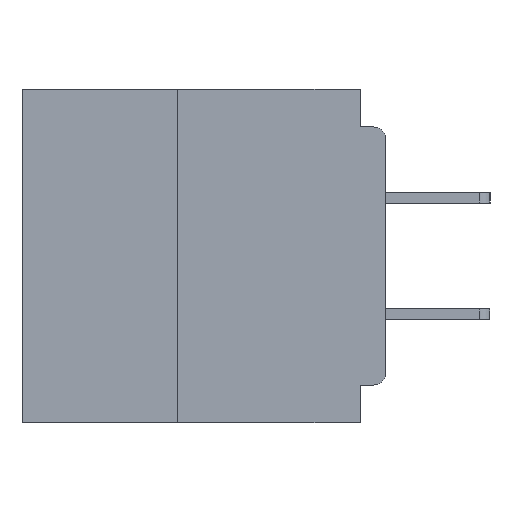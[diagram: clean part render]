
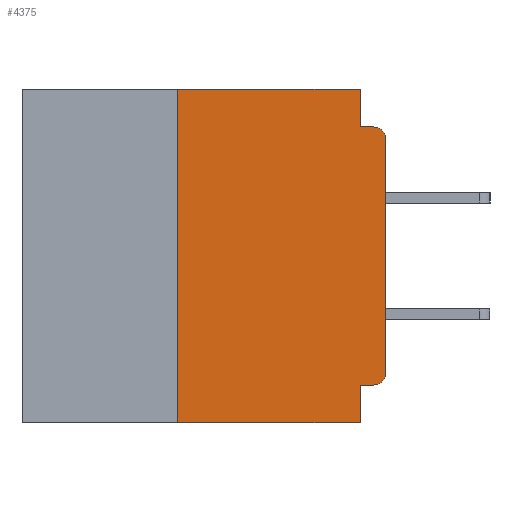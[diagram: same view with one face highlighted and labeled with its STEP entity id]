
A CAD part, left-side view. The second image highlights one B-rep face of the part: STEP entity #4375.
In plain terms, the highlighted planar face has unit normal (-1, 0, 0).
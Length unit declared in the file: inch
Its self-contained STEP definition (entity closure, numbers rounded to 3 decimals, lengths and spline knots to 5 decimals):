
#726 = EDGE_CURVE ( 'NONE', #33710, #32861, #31863, .T. ) ;
#844 = CIRCLE ( 'NONE', #5606, 0.015 ) ;
#1733 = DIRECTION ( 'NONE',  ( 0., -1., 0. ) ) ;
#3978 = CARTESIAN_POINT ( 'NONE',  ( 0., 0.031, 0. ) ) ;
#4185 = VECTOR ( 'NONE', #20784, 39.37008 ) ;
#4375 = ADVANCED_FACE ( 'NONE', ( #26787 ), #51676, .F. ) ;
#4654 = CARTESIAN_POINT ( 'NONE',  ( 0., 0., 0. ) ) ;
#4858 = DIRECTION ( 'NONE',  ( 0., 1., 0. ) ) ;
#5606 = AXIS2_PLACEMENT_3D ( 'NONE', #35649, #9319, #39950 ) ;
#5641 = ORIENTED_EDGE ( 'NONE', *, *, #44179, .F. ) ;
#5864 = CARTESIAN_POINT ( 'NONE',  ( 0., 0.015, -0.045 ) ) ;
#7448 = VERTEX_POINT ( 'NONE', #21349 ) ;
#7575 = CARTESIAN_POINT ( 'NONE',  ( 0., 0.015, -0.06 ) ) ;
#7986 = ORIENTED_EDGE ( 'NONE', *, *, #52729, .F. ) ;
#8077 = VECTOR ( 'NONE', #16363, 39.37008 ) ;
#8867 = VERTEX_POINT ( 'NONE', #40444 ) ;
#9319 = DIRECTION ( 'NONE',  ( -1., 0., 0. ) ) ;
#13557 = LINE ( 'NONE', #39957, #36845 ) ;
#13587 = DIRECTION ( 'NONE',  ( 0., 0., 1. ) ) ;
#13747 = VECTOR ( 'NONE', #1733, 39.37008 ) ;
#14950 = VERTEX_POINT ( 'NONE', #47479 ) ;
#16192 = CARTESIAN_POINT ( 'NONE',  ( 0., 0., -0.045 ) ) ;
#16347 = EDGE_LOOP ( 'NONE', ( #53151, #26699, #54415, #7986, #5641, #36179, #53733, #44092, #44790, #26195 ) ) ;
#16363 = DIRECTION ( 'NONE',  ( 0., -1., 0. ) ) ;
#16460 = CARTESIAN_POINT ( 'NONE',  ( 0., 0.015, -0.355 ) ) ;
#17698 = DIRECTION ( 'NONE',  ( 0., 0., -1. ) ) ;
#18506 = EDGE_CURVE ( 'NONE', #29937, #56159, #13557, .T. ) ;
#19112 = LINE ( 'NONE', #30955, #40934 ) ;
#19751 = LINE ( 'NONE', #34488, #41582 ) ;
#20784 = DIRECTION ( 'NONE',  ( 0., 0., -1. ) ) ;
#21035 = AXIS2_PLACEMENT_3D ( 'NONE', #7575, #27824, #17698 ) ;
#21349 = CARTESIAN_POINT ( 'NONE',  ( 0., 0.031, -0.4 ) ) ;
#23026 = CARTESIAN_POINT ( 'NONE',  ( 0., 0.25, 0. ) ) ;
#23324 = EDGE_CURVE ( 'NONE', #8867, #33710, #36530, .T. ) ;
#24668 = VECTOR ( 'NONE', #38396, 39.37008 ) ;
#26195 = ORIENTED_EDGE ( 'NONE', *, *, #51726, .T. ) ;
#26699 = ORIENTED_EDGE ( 'NONE', *, *, #726, .T. ) ;
#26787 = FACE_OUTER_BOUND ( 'NONE', #16347, .T. ) ;
#27824 = DIRECTION ( 'NONE',  ( -1., 0., 0. ) ) ;
#29469 = EDGE_CURVE ( 'NONE', #56159, #7448, #19112, .T. ) ;
#29937 = VERTEX_POINT ( 'NONE', #16460 ) ;
#30068 = DIRECTION ( 'NONE',  ( 0., 0., -1. ) ) ;
#30955 = CARTESIAN_POINT ( 'NONE',  ( 0., 0.031, -0.4 ) ) ;
#31863 = CIRCLE ( 'NONE', #21035, 0.015 ) ;
#32405 = EDGE_CURVE ( 'NONE', #50454, #7448, #55852, .T. ) ;
#32534 = VERTEX_POINT ( 'NONE', #3978 ) ;
#32861 = VERTEX_POINT ( 'NONE', #5864 ) ;
#33710 = VERTEX_POINT ( 'NONE', #51564 ) ;
#34488 = CARTESIAN_POINT ( 'NONE',  ( 0., 0.25, -0.4 ) ) ;
#35329 = DIRECTION ( 'NONE',  ( 0., 0., -1. ) ) ;
#35649 = CARTESIAN_POINT ( 'NONE',  ( 0., 0.015, -0.34 ) ) ;
#36179 = ORIENTED_EDGE ( 'NONE', *, *, #49793, .F. ) ;
#36285 = LINE ( 'NONE', #16192, #24668 ) ;
#36530 = LINE ( 'NONE', #4654, #45314 ) ;
#36845 = VECTOR ( 'NONE', #4858, 39.37008 ) ;
#38391 = LINE ( 'NONE', #45466, #13747 ) ;
#38396 = DIRECTION ( 'NONE',  ( 0., -1., 0. ) ) ;
#38813 = DIRECTION ( 'NONE',  ( 0., 0., 1. ) ) ;
#39227 = LINE ( 'NONE', #46879, #4185 ) ;
#39950 = DIRECTION ( 'NONE',  ( 0., 0., -1. ) ) ;
#39957 = CARTESIAN_POINT ( 'NONE',  ( 0., 0., -0.355 ) ) ;
#40444 = CARTESIAN_POINT ( 'NONE',  ( 0., 0., -0.34 ) ) ;
#40783 = VERTEX_POINT ( 'NONE', #23026 ) ;
#40934 = VECTOR ( 'NONE', #35329, 39.37008 ) ;
#41582 = VECTOR ( 'NONE', #38813, 39.37008 ) ;
#42526 = CARTESIAN_POINT ( 'NONE',  ( 0., 0.437, -0.4 ) ) ;
#42934 = CARTESIAN_POINT ( 'NONE',  ( 0., 0.437, 0. ) ) ;
#44092 = ORIENTED_EDGE ( 'NONE', *, *, #29469, .F. ) ;
#44179 = EDGE_CURVE ( 'NONE', #40783, #32534, #38391, .T. ) ;
#44790 = ORIENTED_EDGE ( 'NONE', *, *, #18506, .F. ) ;
#44841 = EDGE_CURVE ( 'NONE', #14950, #32861, #36285, .T. ) ;
#45314 = VECTOR ( 'NONE', #13587, 39.37008 ) ;
#45466 = CARTESIAN_POINT ( 'NONE',  ( 0., 0.437, 0. ) ) ;
#46879 = CARTESIAN_POINT ( 'NONE',  ( 0., 0.031, 0. ) ) ;
#47479 = CARTESIAN_POINT ( 'NONE',  ( 0., 0.031, -0.045 ) ) ;
#49793 = EDGE_CURVE ( 'NONE', #50454, #40783, #19751, .T. ) ;
#50454 = VERTEX_POINT ( 'NONE', #52411 ) ;
#51564 = CARTESIAN_POINT ( 'NONE',  ( 0., 0., -0.06 ) ) ;
#51676 = PLANE ( 'NONE',  #54635 ) ;
#51726 = EDGE_CURVE ( 'NONE', #29937, #8867, #844, .T. ) ;
#52411 = CARTESIAN_POINT ( 'NONE',  ( 0., 0.25, -0.4 ) ) ;
#52729 = EDGE_CURVE ( 'NONE', #32534, #14950, #39227, .T. ) ;
#53151 = ORIENTED_EDGE ( 'NONE', *, *, #23324, .T. ) ;
#53733 = ORIENTED_EDGE ( 'NONE', *, *, #32405, .T. ) ;
#54415 = ORIENTED_EDGE ( 'NONE', *, *, #44841, .F. ) ;
#54583 = CARTESIAN_POINT ( 'NONE',  ( 0., 0.031, -0.355 ) ) ;
#54635 = AXIS2_PLACEMENT_3D ( 'NONE', #42934, #55964, #30068 ) ;
#55852 = LINE ( 'NONE', #42526, #8077 ) ;
#55964 = DIRECTION ( 'NONE',  ( 1., 0., 0. ) ) ;
#56159 = VERTEX_POINT ( 'NONE', #54583 ) ;
